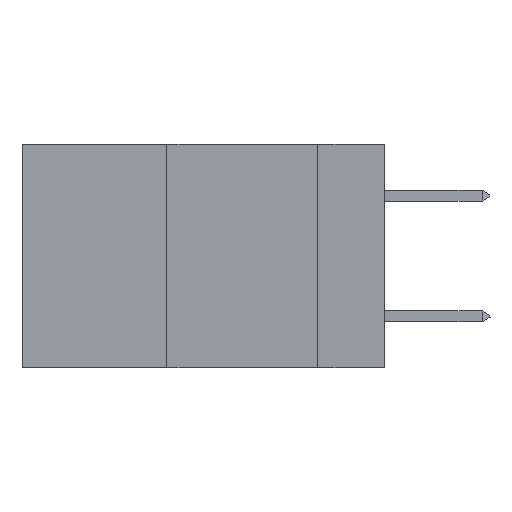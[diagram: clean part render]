
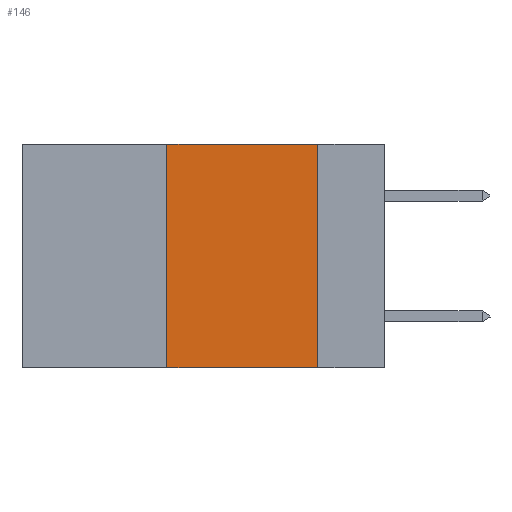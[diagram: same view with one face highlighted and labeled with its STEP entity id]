
A CAD part, left-side view. The second image highlights one B-rep face of the part: STEP entity #146.
In plain terms, the highlighted planar face has unit normal (-1, 0, 0).
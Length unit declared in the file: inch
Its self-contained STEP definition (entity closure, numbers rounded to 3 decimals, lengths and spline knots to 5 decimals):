
#146 = ADVANCED_FACE ( 'NONE', ( #11557 ), #19601, .F. ) ;
#1212 = CARTESIAN_POINT ( 'NONE',  ( 0., 0.6, -0.37 ) ) ;
#1786 = ORIENTED_EDGE ( 'NONE', *, *, #17927, .F. ) ;
#3124 = VECTOR ( 'NONE', #23477, 39.37008 ) ;
#3980 = DIRECTION ( 'NONE',  ( 0., -1., 0. ) ) ;
#4169 = ORIENTED_EDGE ( 'NONE', *, *, #16034, .F. ) ;
#4598 = CARTESIAN_POINT ( 'NONE',  ( 0., 0.6, 0. ) ) ;
#6123 = VECTOR ( 'NONE', #13418, 39.37008 ) ;
#7021 = CARTESIAN_POINT ( 'NONE',  ( 0., 0.11, 0. ) ) ;
#7564 = VERTEX_POINT ( 'NONE', #7021 ) ;
#8304 = LINE ( 'NONE', #14554, #10593 ) ;
#9053 = CARTESIAN_POINT ( 'NONE',  ( 0., 0.6, 0. ) ) ;
#9322 = VERTEX_POINT ( 'NONE', #26956 ) ;
#9784 = VERTEX_POINT ( 'NONE', #23124 ) ;
#10593 = VECTOR ( 'NONE', #14338, 39.37008 ) ;
#11557 = FACE_OUTER_BOUND ( 'NONE', #15004, .T. ) ;
#12720 = LINE ( 'NONE', #18525, #6123 ) ;
#13418 = DIRECTION ( 'NONE',  ( 0., 0., -1. ) ) ;
#14338 = DIRECTION ( 'NONE',  ( 0., 0., 1. ) ) ;
#14554 = CARTESIAN_POINT ( 'NONE',  ( 0., 0.36, 0. ) ) ;
#15004 = EDGE_LOOP ( 'NONE', ( #29475, #1786, #4169, #29854 ) ) ;
#15516 = VECTOR ( 'NONE', #3980, 39.37008 ) ;
#16034 = EDGE_CURVE ( 'NONE', #9322, #9784, #8304, .T. ) ;
#17140 = CARTESIAN_POINT ( 'NONE',  ( 0., 0.11, -0.37 ) ) ;
#17927 = EDGE_CURVE ( 'NONE', #9784, #7564, #24829, .T. ) ;
#18525 = CARTESIAN_POINT ( 'NONE',  ( 0., 0.11, 0. ) ) ;
#18613 = EDGE_CURVE ( 'NONE', #9322, #22474, #30925, .T. ) ;
#19388 = DIRECTION ( 'NONE',  ( 0., 0., -1. ) ) ;
#19601 = PLANE ( 'NONE',  #31705 ) ;
#19973 = EDGE_CURVE ( 'NONE', #7564, #22474, #12720, .T. ) ;
#22273 = DIRECTION ( 'NONE',  ( 1., 0., 0. ) ) ;
#22474 = VERTEX_POINT ( 'NONE', #17140 ) ;
#23124 = CARTESIAN_POINT ( 'NONE',  ( 0., 0.36, 0. ) ) ;
#23477 = DIRECTION ( 'NONE',  ( 0., -1., 0. ) ) ;
#24829 = LINE ( 'NONE', #9053, #15516 ) ;
#26956 = CARTESIAN_POINT ( 'NONE',  ( 0., 0.36, -0.37 ) ) ;
#29475 = ORIENTED_EDGE ( 'NONE', *, *, #19973, .F. ) ;
#29854 = ORIENTED_EDGE ( 'NONE', *, *, #18613, .T. ) ;
#30925 = LINE ( 'NONE', #1212, #3124 ) ;
#31705 = AXIS2_PLACEMENT_3D ( 'NONE', #4598, #22273, #19388 ) ;
